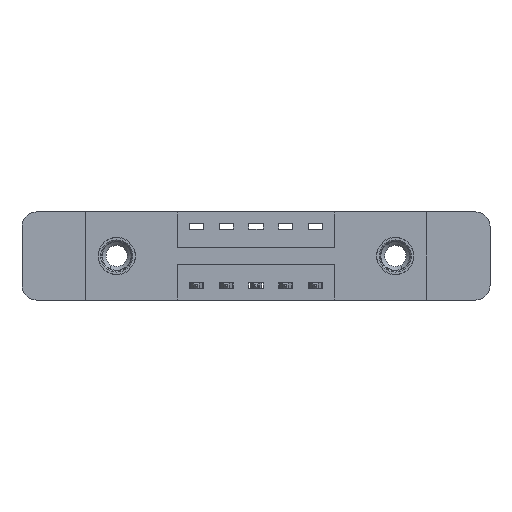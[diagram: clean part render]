
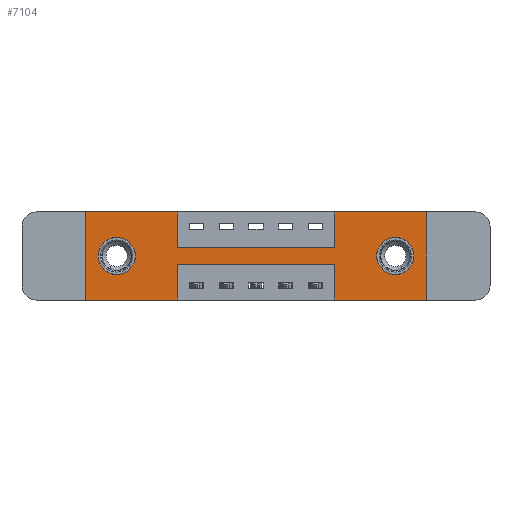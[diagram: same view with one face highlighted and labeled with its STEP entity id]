
A CAD part, front view. The second image highlights one B-rep face of the part: STEP entity #7104.
In plain terms, the highlighted planar face has unit normal (0, -1, 0).
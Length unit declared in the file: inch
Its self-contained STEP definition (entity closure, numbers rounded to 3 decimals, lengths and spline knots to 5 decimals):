
#107 = EDGE_CURVE ( 'NONE', #4284, #314, #9468, .T. ) ;
#300 = LINE ( 'NONE', #12812, #10888 ) ;
#307 = VECTOR ( 'NONE', #5308, 39.37008 ) ;
#314 = VERTEX_POINT ( 'NONE', #7423 ) ;
#346 = EDGE_CURVE ( 'NONE', #12764, #10508, #2997, .T. ) ;
#397 = VERTEX_POINT ( 'NONE', #12863 ) ;
#671 = EDGE_CURVE ( 'NONE', #10961, #5030, #9191, .T. ) ;
#775 = AXIS2_PLACEMENT_3D ( 'NONE', #4731, #2568, #10988 ) ;
#1057 = LINE ( 'NONE', #3214, #307 ) ;
#1464 = CARTESIAN_POINT ( 'NONE',  ( 1.435, 0., 0. ) ) ;
#1538 = VERTEX_POINT ( 'NONE', #11722 ) ;
#1640 = FACE_BOUND ( 'NONE', #12929, .T. ) ;
#1873 = CIRCLE ( 'NONE', #4349, 0.078 ) ;
#2037 = ORIENTED_EDGE ( 'NONE', *, *, #5724, .F. ) ;
#2211 = CARTESIAN_POINT ( 'NONE',  ( 0.3875, 0., -0.15 ) ) ;
#2259 = VECTOR ( 'NONE', #3964, 39.37008 ) ;
#2421 = CARTESIAN_POINT ( 'NONE',  ( 0.3875, 0., -0.15 ) ) ;
#2454 = VECTOR ( 'NONE', #11472, 39.37008 ) ;
#2499 = ORIENTED_EDGE ( 'NONE', *, *, #5441, .F. ) ;
#2512 = CARTESIAN_POINT ( 'NONE',  ( 1.3025, 0., -0.185 ) ) ;
#2568 = DIRECTION ( 'NONE',  ( 0., -1., 0. ) ) ;
#2630 = DIRECTION ( 'NONE',  ( 0., 0., -1. ) ) ;
#2687 = LINE ( 'NONE', #5062, #8782 ) ;
#2737 = ORIENTED_EDGE ( 'NONE', *, *, #346, .T. ) ;
#2997 = CIRCLE ( 'NONE', #7396, 0.078 ) ;
#3214 = CARTESIAN_POINT ( 'NONE',  ( 0., 0., 0. ) ) ;
#3300 = VERTEX_POINT ( 'NONE', #13629 ) ;
#3884 = ORIENTED_EDGE ( 'NONE', *, *, #8607, .F. ) ;
#3964 = DIRECTION ( 'NONE',  ( -1., 0., 0. ) ) ;
#4284 = VERTEX_POINT ( 'NONE', #5548 ) ;
#4349 = AXIS2_PLACEMENT_3D ( 'NONE', #13104, #6890, #10222 ) ;
#4494 = ORIENTED_EDGE ( 'NONE', *, *, #7508, .F. ) ;
#4506 = CIRCLE ( 'NONE', #8018, 0.078 ) ;
#4531 = VERTEX_POINT ( 'NONE', #7674 ) ;
#4613 = LINE ( 'NONE', #12013, #5880 ) ;
#4686 = DIRECTION ( 'NONE',  ( 0., 0., -1. ) ) ;
#4702 = VECTOR ( 'NONE', #10822, 39.37008 ) ;
#4731 = CARTESIAN_POINT ( 'NONE',  ( 0., 0., -0.37 ) ) ;
#4816 = CARTESIAN_POINT ( 'NONE',  ( 1.3025, 0., -0.185 ) ) ;
#4936 = FACE_BOUND ( 'NONE', #6690, .T. ) ;
#5030 = VERTEX_POINT ( 'NONE', #10195 ) ;
#5062 = CARTESIAN_POINT ( 'NONE',  ( 0., 0., 0. ) ) ;
#5255 = CARTESIAN_POINT ( 'NONE',  ( 0., 0., 0. ) ) ;
#5298 = VERTEX_POINT ( 'NONE', #12622 ) ;
#5308 = DIRECTION ( 'NONE',  ( 0., 0., 1. ) ) ;
#5341 = CARTESIAN_POINT ( 'NONE',  ( 0.1325, 0., -0.263 ) ) ;
#5393 = DIRECTION ( 'NONE',  ( 0., 0., -1. ) ) ;
#5441 = EDGE_CURVE ( 'NONE', #12993, #4531, #11344, .T. ) ;
#5476 = VERTEX_POINT ( 'NONE', #12217 ) ;
#5548 = CARTESIAN_POINT ( 'NONE',  ( 1.0475, 0., 0. ) ) ;
#5693 = DIRECTION ( 'NONE',  ( 0., 0., -1. ) ) ;
#5724 = EDGE_CURVE ( 'NONE', #5298, #12825, #4613, .T. ) ;
#5761 = ORIENTED_EDGE ( 'NONE', *, *, #10062, .F. ) ;
#5880 = VECTOR ( 'NONE', #8818, 39.37008 ) ;
#5885 = VECTOR ( 'NONE', #12976, 39.37008 ) ;
#6355 = LINE ( 'NONE', #6431, #12991 ) ;
#6422 = ORIENTED_EDGE ( 'NONE', *, *, #13239, .F. ) ;
#6431 = CARTESIAN_POINT ( 'NONE',  ( 0.3875, 0., 0. ) ) ;
#6628 = EDGE_CURVE ( 'NONE', #11975, #8421, #12787, .T. ) ;
#6690 = EDGE_LOOP ( 'NONE', ( #12294, #2737 ) ) ;
#6692 = CARTESIAN_POINT ( 'NONE',  ( 1.0475, 0., 0. ) ) ;
#6714 = CARTESIAN_POINT ( 'NONE',  ( 0.3875, 0., -0.37 ) ) ;
#6890 = DIRECTION ( 'NONE',  ( 0., 1., 0. ) ) ;
#6977 = CARTESIAN_POINT ( 'NONE',  ( 1.0475, 0., -0.15 ) ) ;
#7104 = ADVANCED_FACE ( 'NONE', ( #4936, #1640, #12218 ), #8867, .T. ) ;
#7334 = ORIENTED_EDGE ( 'NONE', *, *, #7803, .F. ) ;
#7383 = EDGE_CURVE ( 'NONE', #397, #11975, #6355, .T. ) ;
#7396 = AXIS2_PLACEMENT_3D ( 'NONE', #2512, #8748, #4686 ) ;
#7423 = CARTESIAN_POINT ( 'NONE',  ( 1.435, 0., 0. ) ) ;
#7447 = ORIENTED_EDGE ( 'NONE', *, *, #12378, .T. ) ;
#7508 = EDGE_CURVE ( 'NONE', #3300, #12993, #13276, .T. ) ;
#7513 = DIRECTION ( 'NONE',  ( -1., 0., 0. ) ) ;
#7674 = CARTESIAN_POINT ( 'NONE',  ( 0., 0., -0.37 ) ) ;
#7803 = EDGE_CURVE ( 'NONE', #8421, #4284, #11894, .T. ) ;
#7840 = LINE ( 'NONE', #13195, #12568 ) ;
#7860 = VECTOR ( 'NONE', #5693, 39.37008 ) ;
#8012 = CARTESIAN_POINT ( 'NONE',  ( 0., 0., -0.37 ) ) ;
#8018 = AXIS2_PLACEMENT_3D ( 'NONE', #4816, #13061, #10809 ) ;
#8421 = VERTEX_POINT ( 'NONE', #6977 ) ;
#8601 = LINE ( 'NONE', #1464, #7860 ) ;
#8607 = EDGE_CURVE ( 'NONE', #1538, #5298, #7840, .T. ) ;
#8748 = DIRECTION ( 'NONE',  ( 0., 1., 0. ) ) ;
#8782 = VECTOR ( 'NONE', #11181, 39.37008 ) ;
#8818 = DIRECTION ( 'NONE',  ( 0., 0., 1. ) ) ;
#8867 = PLANE ( 'NONE',  #775 ) ;
#9013 = EDGE_CURVE ( 'NONE', #12825, #3300, #300, .T. ) ;
#9069 = DIRECTION ( 'NONE',  ( 0., 1., 0. ) ) ;
#9191 = CIRCLE ( 'NONE', #12531, 0.078 ) ;
#9233 = CARTESIAN_POINT ( 'NONE',  ( 1.3025, 0., -0.263 ) ) ;
#9238 = EDGE_CURVE ( 'NONE', #10508, #12764, #4506, .T. ) ;
#9468 = LINE ( 'NONE', #5255, #2454 ) ;
#9970 = CARTESIAN_POINT ( 'NONE',  ( 0.3875, 0., -0.37 ) ) ;
#10062 = EDGE_CURVE ( 'NONE', #4531, #5476, #1057, .T. ) ;
#10195 = CARTESIAN_POINT ( 'NONE',  ( 0.1325, 0., -0.107 ) ) ;
#10222 = DIRECTION ( 'NONE',  ( 0., 0., 1. ) ) ;
#10432 = EDGE_LOOP ( 'NONE', ( #4494, #13226, #2037, #3884, #13145, #10604, #7334, #10918, #11338, #6422, #5761, #2499 ) ) ;
#10508 = VERTEX_POINT ( 'NONE', #12201 ) ;
#10596 = VECTOR ( 'NONE', #2630, 39.37008 ) ;
#10604 = ORIENTED_EDGE ( 'NONE', *, *, #107, .F. ) ;
#10809 = DIRECTION ( 'NONE',  ( 0., 0., -1. ) ) ;
#10822 = DIRECTION ( 'NONE',  ( 0., 0., 1. ) ) ;
#10888 = VECTOR ( 'NONE', #7513, 39.37008 ) ;
#10918 = ORIENTED_EDGE ( 'NONE', *, *, #6628, .F. ) ;
#10961 = VERTEX_POINT ( 'NONE', #5341 ) ;
#10979 = CARTESIAN_POINT ( 'NONE',  ( 0.1325, 0., -0.185 ) ) ;
#10988 = DIRECTION ( 'NONE',  ( 0., 0., -1. ) ) ;
#11089 = DIRECTION ( 'NONE',  ( -1., 0., 0. ) ) ;
#11181 = DIRECTION ( 'NONE',  ( 1., 0., 0. ) ) ;
#11338 = ORIENTED_EDGE ( 'NONE', *, *, #7383, .F. ) ;
#11344 = LINE ( 'NONE', #8012, #2259 ) ;
#11472 = DIRECTION ( 'NONE',  ( 1., 0., 0. ) ) ;
#11722 = CARTESIAN_POINT ( 'NONE',  ( 1.435, 0., -0.37 ) ) ;
#11790 = ORIENTED_EDGE ( 'NONE', *, *, #671, .T. ) ;
#11894 = LINE ( 'NONE', #6692, #4702 ) ;
#11975 = VERTEX_POINT ( 'NONE', #2421 ) ;
#12013 = CARTESIAN_POINT ( 'NONE',  ( 1.0475, 0., -0.37 ) ) ;
#12201 = CARTESIAN_POINT ( 'NONE',  ( 1.3025, 0., -0.107 ) ) ;
#12209 = EDGE_CURVE ( 'NONE', #314, #1538, #8601, .T. ) ;
#12217 = CARTESIAN_POINT ( 'NONE',  ( 0., 0., 0. ) ) ;
#12218 = FACE_OUTER_BOUND ( 'NONE', #10432, .T. ) ;
#12294 = ORIENTED_EDGE ( 'NONE', *, *, #9238, .T. ) ;
#12358 = CARTESIAN_POINT ( 'NONE',  ( 1.0475, 0., -0.22 ) ) ;
#12378 = EDGE_CURVE ( 'NONE', #5030, #10961, #1873, .T. ) ;
#12531 = AXIS2_PLACEMENT_3D ( 'NONE', #10979, #9069, #13028 ) ;
#12568 = VECTOR ( 'NONE', #11089, 39.37008 ) ;
#12622 = CARTESIAN_POINT ( 'NONE',  ( 1.0475, 0., -0.37 ) ) ;
#12764 = VERTEX_POINT ( 'NONE', #9233 ) ;
#12787 = LINE ( 'NONE', #2211, #5885 ) ;
#12812 = CARTESIAN_POINT ( 'NONE',  ( 0.3875, 0., -0.22 ) ) ;
#12825 = VERTEX_POINT ( 'NONE', #12358 ) ;
#12863 = CARTESIAN_POINT ( 'NONE',  ( 0.3875, 0., 0. ) ) ;
#12929 = EDGE_LOOP ( 'NONE', ( #7447, #11790 ) ) ;
#12976 = DIRECTION ( 'NONE',  ( 1., 0., 0. ) ) ;
#12991 = VECTOR ( 'NONE', #5393, 39.37008 ) ;
#12993 = VERTEX_POINT ( 'NONE', #9970 ) ;
#13028 = DIRECTION ( 'NONE',  ( 0., 0., 1. ) ) ;
#13061 = DIRECTION ( 'NONE',  ( 0., 1., 0. ) ) ;
#13104 = CARTESIAN_POINT ( 'NONE',  ( 0.1325, 0., -0.185 ) ) ;
#13145 = ORIENTED_EDGE ( 'NONE', *, *, #12209, .F. ) ;
#13195 = CARTESIAN_POINT ( 'NONE',  ( 0., 0., -0.37 ) ) ;
#13226 = ORIENTED_EDGE ( 'NONE', *, *, #9013, .F. ) ;
#13239 = EDGE_CURVE ( 'NONE', #5476, #397, #2687, .T. ) ;
#13276 = LINE ( 'NONE', #6714, #10596 ) ;
#13629 = CARTESIAN_POINT ( 'NONE',  ( 0.3875, 0., -0.22 ) ) ;
